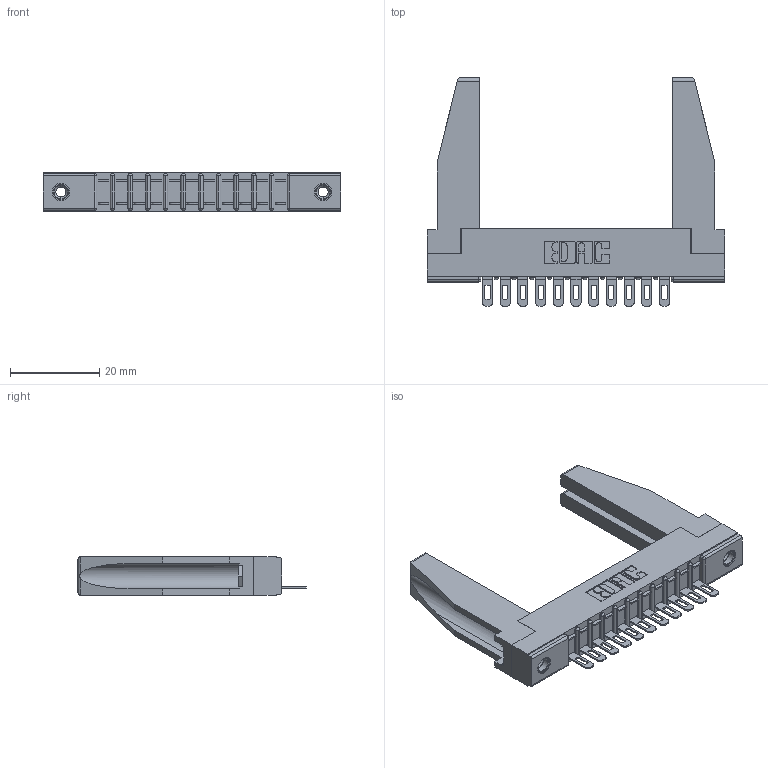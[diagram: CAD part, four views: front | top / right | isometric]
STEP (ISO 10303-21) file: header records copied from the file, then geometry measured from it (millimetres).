
FILE_DESCRIPTION (( 'STEP AP203' ), '1' );
FILE_NAME ('357-011-401-178.STEP', '2020-09-30T09:52:44', ( '' ), ( '' ), 'SwSTEP 2.0', 'SolidWorks 2020', '' );
FILE_SCHEMA (( 'CONFIG_CONTROL_DESIGN' ));
Length unit declared in the file: inch
Products named in the file (5): 307-220-078; 307-290-002_501; 307 Part_.156 Dia Mounting Holes; 357-011-401-178; 345-250-001_345-250-001-102
Assembly tree (16 placements, depth 2):
  357-011-401-178
    307 Part_.156 Dia Mounting Holes
    307-290-002_501  x11
    307-220-078  x2
    345-250-001_345-250-001-102  x2
Bounding box: 66.6 x 51.13 x 8.71 mm (x, y, z)
Volume: 8393.9 mm3; surface area: 11287 mm2
Topology: 16 solids, 16 shells, 1096 faces, 3271 edges, 2138 vertices
Faces by surface type: plane 638, cylinder 418, sphere 24, cone 12, torus 4
Entity records: 16485 total; most frequent: CARTESIAN_POINT 2774, ORIENTED_EDGE 2720, DIRECTION 2670, EDGE_CURVE 1360, VECTOR 1026, LINE 1026, VERTEX_POINT 884, AXIS2_PLACEMENT_3D 822
